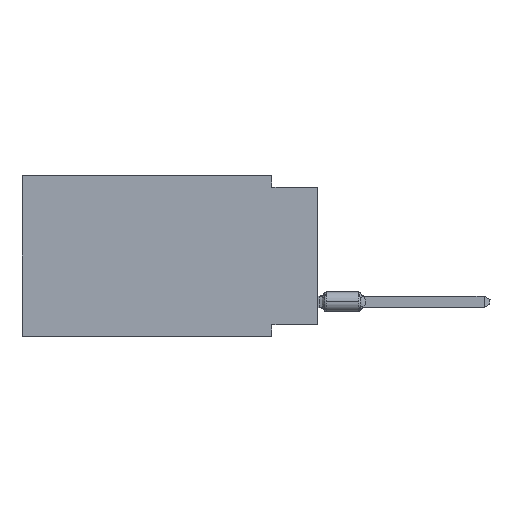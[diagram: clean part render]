
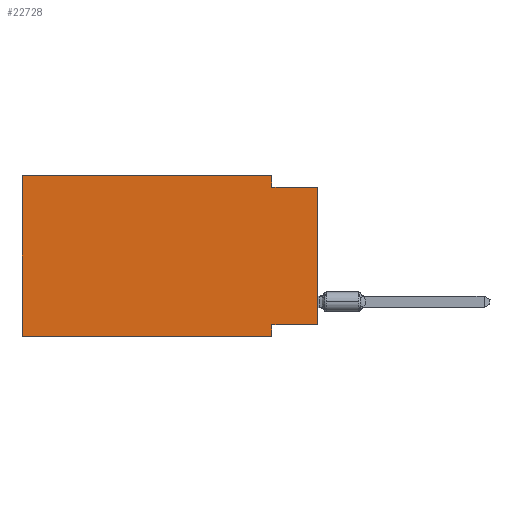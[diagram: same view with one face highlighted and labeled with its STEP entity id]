
A CAD part, left-side view. The second image highlights one B-rep face of the part: STEP entity #22728.
In plain terms, the highlighted planar face has unit normal (-1, 0, 0).
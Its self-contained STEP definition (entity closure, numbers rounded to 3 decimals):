
#208 = CARTESIAN_POINT ( 'NONE',  ( 0., 0., -8.255 ) ) ;
#723 = CARTESIAN_POINT ( 'NONE',  ( 0., 0., -0.635 ) ) ;
#1982 = DIRECTION ( 'NONE',  ( 0., 0., 1. ) ) ;
#2005 = VECTOR ( 'NONE', #27624, 1000. ) ;
#2117 = CARTESIAN_POINT ( 'NONE',  ( 0., 2.54, 0. ) ) ;
#2274 = VECTOR ( 'NONE', #7766, 1000. ) ;
#3076 = AXIS2_PLACEMENT_3D ( 'NONE', #11664, #4798, #26071 ) ;
#4798 = DIRECTION ( 'NONE',  ( 1., 0., 0. ) ) ;
#5227 = EDGE_CURVE ( 'NONE', #15354, #44338, #37352, .T. ) ;
#7494 = DIRECTION ( 'NONE',  ( 0., 1., 0. ) ) ;
#7766 = DIRECTION ( 'NONE',  ( 0., -1., 0. ) ) ;
#7939 = ORIENTED_EDGE ( 'NONE', *, *, #31603, .T. ) ;
#8418 = ORIENTED_EDGE ( 'NONE', *, *, #36642, .F. ) ;
#8726 = LINE ( 'NONE', #2117, #38562 ) ;
#9451 = VECTOR ( 'NONE', #14663, 1000. ) ;
#9641 = VECTOR ( 'NONE', #1982, 1000. ) ;
#9676 = EDGE_CURVE ( 'NONE', #46310, #25959, #15787, .T. ) ;
#10198 = CARTESIAN_POINT ( 'NONE',  ( 0., 0., -0.635 ) ) ;
#10858 = CARTESIAN_POINT ( 'NONE',  ( 0., 2.54, -8.255 ) ) ;
#11664 = CARTESIAN_POINT ( 'NONE',  ( 0., 16.383, 0. ) ) ;
#13282 = EDGE_CURVE ( 'NONE', #17689, #46299, #25068, .T. ) ;
#13573 = DIRECTION ( 'NONE',  ( 0., 0., 1. ) ) ;
#13976 = ORIENTED_EDGE ( 'NONE', *, *, #5227, .T. ) ;
#14663 = DIRECTION ( 'NONE',  ( 0., -1., 0. ) ) ;
#14786 = EDGE_LOOP ( 'NONE', ( #7939, #45690, #8418, #19634, #41787, #13976, #44185, #27266 ) ) ;
#15354 = VERTEX_POINT ( 'NONE', #15709 ) ;
#15709 = CARTESIAN_POINT ( 'NONE',  ( 0., 16.383, -8.89 ) ) ;
#15787 = LINE ( 'NONE', #723, #2274 ) ;
#16293 = LINE ( 'NONE', #45767, #2005 ) ;
#17689 = VERTEX_POINT ( 'NONE', #28352 ) ;
#17888 = LINE ( 'NONE', #208, #20341 ) ;
#19634 = ORIENTED_EDGE ( 'NONE', *, *, #13282, .F. ) ;
#19642 = EDGE_CURVE ( 'NONE', #43097, #27877, #17888, .T. ) ;
#20341 = VECTOR ( 'NONE', #7494, 1000. ) ;
#22525 = PLANE ( 'NONE',  #3076 ) ;
#22728 = ADVANCED_FACE ( 'NONE', ( #29616 ), #22525, .F. ) ;
#25068 = LINE ( 'NONE', #39451, #9451 ) ;
#25959 = VERTEX_POINT ( 'NONE', #10198 ) ;
#26071 = DIRECTION ( 'NONE',  ( 0., 0., -1. ) ) ;
#26188 = CARTESIAN_POINT ( 'NONE',  ( 0., 2.54, -8.89 ) ) ;
#26964 = VECTOR ( 'NONE', #13573, 1000. ) ;
#27266 = ORIENTED_EDGE ( 'NONE', *, *, #19642, .F. ) ;
#27624 = DIRECTION ( 'NONE',  ( 0., 0., -1. ) ) ;
#27877 = VERTEX_POINT ( 'NONE', #10858 ) ;
#28352 = CARTESIAN_POINT ( 'NONE',  ( 0., 16.383, 0. ) ) ;
#29616 = FACE_OUTER_BOUND ( 'NONE', #14786, .T. ) ;
#29999 = DIRECTION ( 'NONE',  ( 0., 0., -1. ) ) ;
#30658 = VECTOR ( 'NONE', #42739, 1000. ) ;
#31603 = EDGE_CURVE ( 'NONE', #43097, #25959, #35269, .T. ) ;
#35016 = CARTESIAN_POINT ( 'NONE',  ( 0., 16.383, 0. ) ) ;
#35269 = LINE ( 'NONE', #45885, #26964 ) ;
#35759 = CARTESIAN_POINT ( 'NONE',  ( 0., 2.54, 0. ) ) ;
#36642 = EDGE_CURVE ( 'NONE', #46299, #46310, #8726, .T. ) ;
#37063 = CARTESIAN_POINT ( 'NONE',  ( 0., 0., -8.255 ) ) ;
#37352 = LINE ( 'NONE', #38742, #30658 ) ;
#38562 = VECTOR ( 'NONE', #29999, 1000. ) ;
#38742 = CARTESIAN_POINT ( 'NONE',  ( 0., 16.383, -8.89 ) ) ;
#39313 = CARTESIAN_POINT ( 'NONE',  ( 0., 2.54, -0.635 ) ) ;
#39451 = CARTESIAN_POINT ( 'NONE',  ( 0., 16.383, 0. ) ) ;
#41787 = ORIENTED_EDGE ( 'NONE', *, *, #42514, .F. ) ;
#42514 = EDGE_CURVE ( 'NONE', #15354, #17689, #45618, .T. ) ;
#42739 = DIRECTION ( 'NONE',  ( 0., -1., 0. ) ) ;
#43097 = VERTEX_POINT ( 'NONE', #37063 ) ;
#44185 = ORIENTED_EDGE ( 'NONE', *, *, #45903, .F. ) ;
#44338 = VERTEX_POINT ( 'NONE', #26188 ) ;
#45618 = LINE ( 'NONE', #35016, #9641 ) ;
#45690 = ORIENTED_EDGE ( 'NONE', *, *, #9676, .F. ) ;
#45767 = CARTESIAN_POINT ( 'NONE',  ( 0., 2.54, -8.89 ) ) ;
#45885 = CARTESIAN_POINT ( 'NONE',  ( 0., 0., 0. ) ) ;
#45903 = EDGE_CURVE ( 'NONE', #27877, #44338, #16293, .T. ) ;
#46299 = VERTEX_POINT ( 'NONE', #35759 ) ;
#46310 = VERTEX_POINT ( 'NONE', #39313 ) ;
